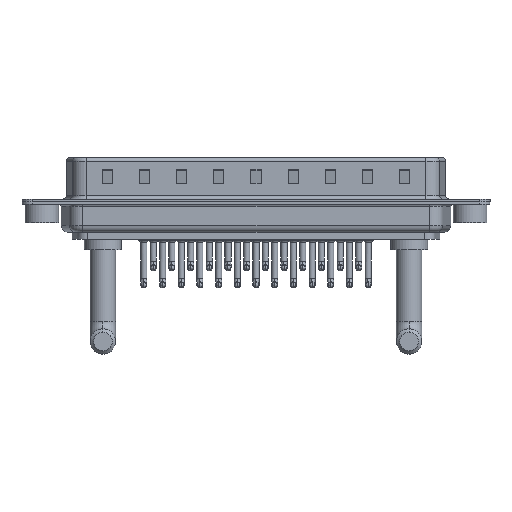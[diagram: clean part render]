
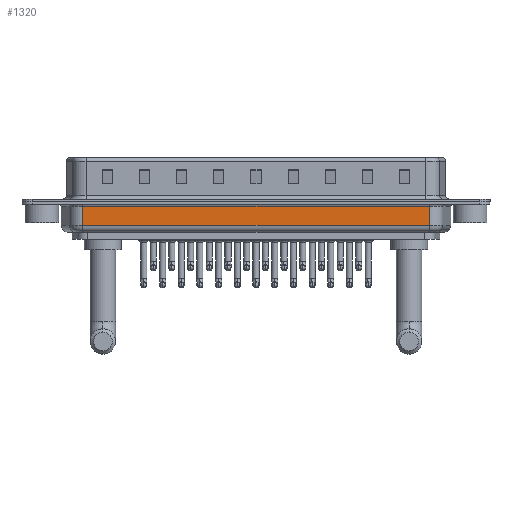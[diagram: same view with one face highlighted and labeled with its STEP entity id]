
A CAD part, front view. The second image highlights one B-rep face of the part: STEP entity #1320.
In plain terms, the highlighted planar face has unit normal (0, -1, 0).
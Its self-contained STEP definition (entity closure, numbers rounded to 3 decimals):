
#1320 = ADVANCED_FACE ( 'NONE', ( #3252 ), #12078, .F. ) ;
#2300 = CARTESIAN_POINT ( 'NONE',  ( 6.031, -5.35, -0.65 ) ) ;
#3252 = FACE_OUTER_BOUND ( 'NONE', #13957, .T. ) ;
#4347 = VERTEX_POINT ( 'NONE', #25538 ) ;
#4664 = ORIENTED_EDGE ( 'NONE', *, *, #18717, .T. ) ;
#5253 = EDGE_CURVE ( 'NONE', #4347, #19946, #21695, .T. ) ;
#5675 = ORIENTED_EDGE ( 'NONE', *, *, #23636, .T. ) ;
#8218 = DIRECTION ( 'NONE',  ( 0., 0., 1. ) ) ;
#8757 = DIRECTION ( 'NONE',  ( 0., 0., 1. ) ) ;
#9078 = ORIENTED_EDGE ( 'NONE', *, *, #14340, .T. ) ;
#10006 = ORIENTED_EDGE ( 'NONE', *, *, #5253, .F. ) ;
#10928 = LINE ( 'NONE', #22353, #15047 ) ;
#12078 = PLANE ( 'NONE',  #19794 ) ;
#12455 = VECTOR ( 'NONE', #21345, 1000. ) ;
#13957 = EDGE_LOOP ( 'NONE', ( #10006, #5675, #4664, #9078 ) ) ;
#14340 = EDGE_CURVE ( 'NONE', #19098, #19946, #22118, .T. ) ;
#15047 = VECTOR ( 'NONE', #8757, 1000. ) ;
#16746 = VECTOR ( 'NONE', #22395, 1000. ) ;
#17572 = LINE ( 'NONE', #27956, #12455 ) ;
#18499 = VERTEX_POINT ( 'NONE', #23797 ) ;
#18717 = EDGE_CURVE ( 'NONE', #18499, #19098, #10928, .T. ) ;
#18726 = DIRECTION ( 'NONE',  ( 0., 1., 0. ) ) ;
#18874 = DIRECTION ( 'NONE',  ( -1., 0., 0. ) ) ;
#19098 = VERTEX_POINT ( 'NONE', #19879 ) ;
#19794 = AXIS2_PLACEMENT_3D ( 'NONE', #20912, #18726, #18874 ) ;
#19879 = CARTESIAN_POINT ( 'NONE',  ( 57.469, -5.35, -0.65 ) ) ;
#19946 = VERTEX_POINT ( 'NONE', #24253 ) ;
#20912 = CARTESIAN_POINT ( 'NONE',  ( 6.031, -5.35, -4.5 ) ) ;
#21345 = DIRECTION ( 'NONE',  ( 1., 0., 0. ) ) ;
#21695 = LINE ( 'NONE', #28026, #26788 ) ;
#22118 = LINE ( 'NONE', #2300, #16746 ) ;
#22353 = CARTESIAN_POINT ( 'NONE',  ( 57.469, -5.35, -4.5 ) ) ;
#22395 = DIRECTION ( 'NONE',  ( -1., 0., 0. ) ) ;
#23636 = EDGE_CURVE ( 'NONE', #4347, #18499, #17572, .T. ) ;
#23797 = CARTESIAN_POINT ( 'NONE',  ( 57.469, -5.35, -3.5 ) ) ;
#24253 = CARTESIAN_POINT ( 'NONE',  ( 6.031, -5.35, -0.65 ) ) ;
#25538 = CARTESIAN_POINT ( 'NONE',  ( 6.031, -5.35, -3.5 ) ) ;
#26788 = VECTOR ( 'NONE', #8218, 1000. ) ;
#27956 = CARTESIAN_POINT ( 'NONE',  ( 6.031, -5.35, -3.5 ) ) ;
#28026 = CARTESIAN_POINT ( 'NONE',  ( 6.031, -5.35, -4.5 ) ) ;
